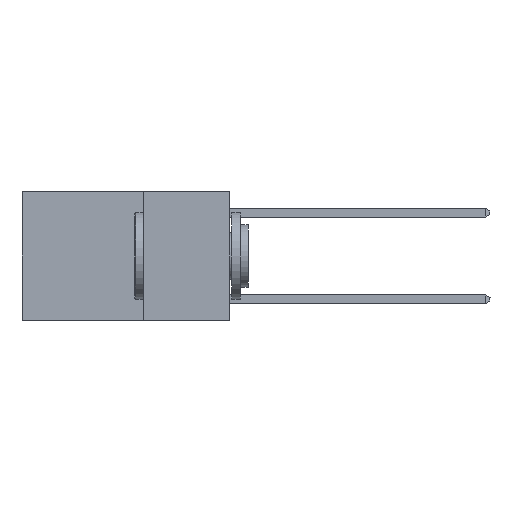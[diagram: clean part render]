
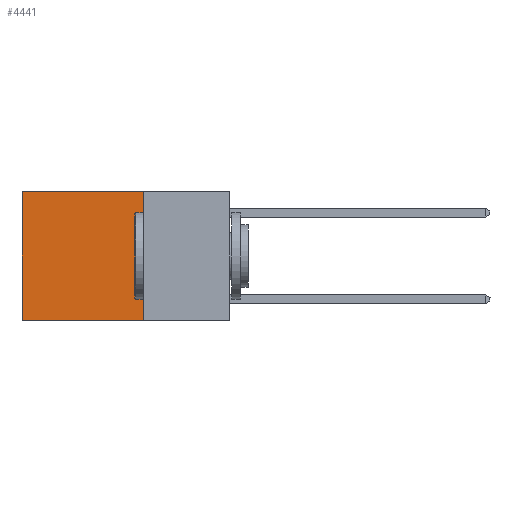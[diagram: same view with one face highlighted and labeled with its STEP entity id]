
A CAD part, left-side view. The second image highlights one B-rep face of the part: STEP entity #4441.
In plain terms, the highlighted planar face has unit normal (-1, 0, 0).
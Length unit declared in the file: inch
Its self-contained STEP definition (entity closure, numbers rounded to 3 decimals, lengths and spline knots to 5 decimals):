
#1879 = EDGE_CURVE ( 'NONE', #18720, #20274, #4253, .T. ) ;
#1985 = EDGE_CURVE ( 'NONE', #10660, #12354, #20988, .T. ) ;
#2585 = VECTOR ( 'NONE', #2886, 39.37008 ) ;
#2886 = DIRECTION ( 'NONE',  ( 0., 0., -1. ) ) ;
#3088 = CARTESIAN_POINT ( 'NONE',  ( 0.2625, 0.25, 0. ) ) ;
#3694 = LINE ( 'NONE', #18272, #16937 ) ;
#4193 = CARTESIAN_POINT ( 'NONE',  ( 0.2625, 0.25, 0. ) ) ;
#4253 = LINE ( 'NONE', #5335, #18555 ) ;
#4441 = ADVANCED_FACE ( 'NONE', ( #19019 ), #21386, .F. ) ;
#5328 = DIRECTION ( 'NONE',  ( 0., 0., -1. ) ) ;
#5335 = CARTESIAN_POINT ( 'NONE',  ( 0.2625, 0.6, 0. ) ) ;
#5510 = CARTESIAN_POINT ( 'NONE',  ( 0.2625, 0.25, -0.37 ) ) ;
#5613 = ORIENTED_EDGE ( 'NONE', *, *, #1985, .F. ) ;
#7148 = CARTESIAN_POINT ( 'NONE',  ( 0.2625, 0.25, -0.37 ) ) ;
#7689 = DIRECTION ( 'NONE',  ( 1., 0., 0. ) ) ;
#7708 = CARTESIAN_POINT ( 'NONE',  ( 0.2625, 0.6, -0.37 ) ) ;
#7806 = CARTESIAN_POINT ( 'NONE',  ( 0.2625, 0.25, 0. ) ) ;
#10280 = VECTOR ( 'NONE', #13925, 39.37008 ) ;
#10660 = VERTEX_POINT ( 'NONE', #7806 ) ;
#11131 = EDGE_LOOP ( 'NONE', ( #19069, #19152, #5613, #18354 ) ) ;
#12354 = VERTEX_POINT ( 'NONE', #5510 ) ;
#13925 = DIRECTION ( 'NONE',  ( 0., 1., 0. ) ) ;
#16357 = EDGE_CURVE ( 'NONE', #12354, #20274, #18893, .T. ) ;
#16937 = VECTOR ( 'NONE', #20001, 39.37008 ) ;
#18272 = CARTESIAN_POINT ( 'NONE',  ( 0.2625, 0.25, 0. ) ) ;
#18354 = ORIENTED_EDGE ( 'NONE', *, *, #19666, .T. ) ;
#18555 = VECTOR ( 'NONE', #5328, 39.37008 ) ;
#18720 = VERTEX_POINT ( 'NONE', #21014 ) ;
#18893 = LINE ( 'NONE', #7148, #10280 ) ;
#19019 = FACE_OUTER_BOUND ( 'NONE', #11131, .T. ) ;
#19069 = ORIENTED_EDGE ( 'NONE', *, *, #1879, .T. ) ;
#19152 = ORIENTED_EDGE ( 'NONE', *, *, #16357, .F. ) ;
#19666 = EDGE_CURVE ( 'NONE', #10660, #18720, #3694, .T. ) ;
#19741 = DIRECTION ( 'NONE',  ( 0., 0., -1. ) ) ;
#20001 = DIRECTION ( 'NONE',  ( 0., 1., 0. ) ) ;
#20274 = VERTEX_POINT ( 'NONE', #7708 ) ;
#20988 = LINE ( 'NONE', #3088, #2585 ) ;
#21014 = CARTESIAN_POINT ( 'NONE',  ( 0.2625, 0.6, 0. ) ) ;
#21386 = PLANE ( 'NONE',  #21953 ) ;
#21953 = AXIS2_PLACEMENT_3D ( 'NONE', #4193, #7689, #19741 ) ;
